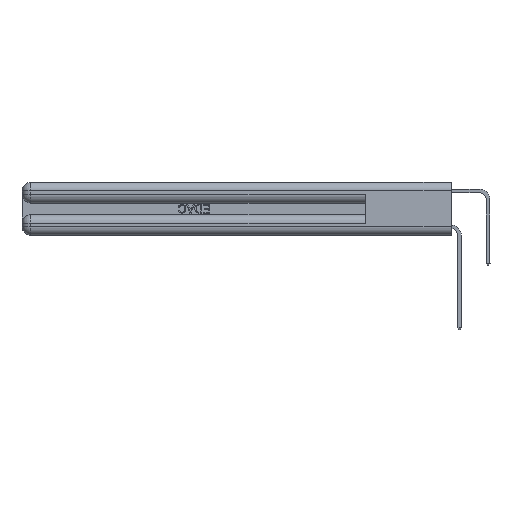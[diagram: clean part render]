
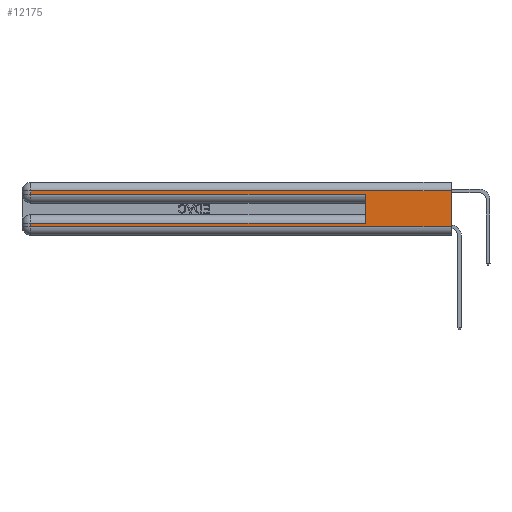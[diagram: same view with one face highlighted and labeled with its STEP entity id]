
A CAD part, left-side view. The second image highlights one B-rep face of the part: STEP entity #12175.
In plain terms, the highlighted planar face has unit normal (-1, 0, 0).
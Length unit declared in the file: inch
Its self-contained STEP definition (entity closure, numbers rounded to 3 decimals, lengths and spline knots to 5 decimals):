
#326 = CARTESIAN_POINT ( 'NONE',  ( 0., 0., 0.31 ) ) ;
#1134 = DIRECTION ( 'NONE',  ( 0., 1., 0. ) ) ;
#1836 = DIRECTION ( 'NONE',  ( 1., 0., 0. ) ) ;
#1907 = CARTESIAN_POINT ( 'NONE',  ( 0., 0., 0.285 ) ) ;
#2095 = DIRECTION ( 'NONE',  ( 0., -1., 0. ) ) ;
#2141 = EDGE_CURVE ( 'NONE', #10791, #7032, #10355, .T. ) ;
#2217 = DIRECTION ( 'NONE',  ( 0., 0., -1. ) ) ;
#2990 = EDGE_CURVE ( 'NONE', #7032, #5058, #13980, .T. ) ;
#3589 = VECTOR ( 'NONE', #2095, 39.37008 ) ;
#4436 = LINE ( 'NONE', #5590, #25466 ) ;
#4993 = DIRECTION ( 'NONE',  ( 0., 1., 0. ) ) ;
#5058 = VERTEX_POINT ( 'NONE', #28188 ) ;
#5516 = CARTESIAN_POINT ( 'NONE',  ( 0., 2.94, 0.31 ) ) ;
#5590 = CARTESIAN_POINT ( 'NONE',  ( 0., 0., 0.37 ) ) ;
#6096 = VECTOR ( 'NONE', #16822, 39.37008 ) ;
#6223 = CARTESIAN_POINT ( 'NONE',  ( 0., 0., 0.085 ) ) ;
#6437 = CARTESIAN_POINT ( 'NONE',  ( 0., 2.94, 0.37 ) ) ;
#7032 = VERTEX_POINT ( 'NONE', #15955 ) ;
#7646 = EDGE_CURVE ( 'NONE', #36003, #35059, #4436, .T. ) ;
#8826 = VERTEX_POINT ( 'NONE', #36131 ) ;
#9264 = AXIS2_PLACEMENT_3D ( 'NONE', #37642, #1836, #2217 ) ;
#10306 = EDGE_CURVE ( 'NONE', #36003, #10791, #22664, .T. ) ;
#10355 = LINE ( 'NONE', #13095, #13495 ) ;
#10791 = VERTEX_POINT ( 'NONE', #5516 ) ;
#11388 = LINE ( 'NONE', #37844, #6096 ) ;
#11722 = DIRECTION ( 'NONE',  ( 0., 0., -1. ) ) ;
#11881 = ORIENTED_EDGE ( 'NONE', *, *, #12666, .T. ) ;
#11940 = ORIENTED_EDGE ( 'NONE', *, *, #2990, .T. ) ;
#12175 = ADVANCED_FACE ( 'NONE', ( #31602 ), #37827, .F. ) ;
#12250 = ORIENTED_EDGE ( 'NONE', *, *, #2141, .T. ) ;
#12666 = EDGE_CURVE ( 'NONE', #25055, #29260, #32144, .T. ) ;
#13095 = CARTESIAN_POINT ( 'NONE',  ( 0., 2.94, 0.37 ) ) ;
#13495 = VECTOR ( 'NONE', #28443, 39.37008 ) ;
#13626 = VECTOR ( 'NONE', #11722, 39.37008 ) ;
#13885 = ORIENTED_EDGE ( 'NONE', *, *, #32631, .F. ) ;
#13980 = LINE ( 'NONE', #1907, #3589 ) ;
#15031 = ORIENTED_EDGE ( 'NONE', *, *, #7646, .F. ) ;
#15081 = ORIENTED_EDGE ( 'NONE', *, *, #21489, .T. ) ;
#15357 = LINE ( 'NONE', #6223, #29559 ) ;
#15955 = CARTESIAN_POINT ( 'NONE',  ( 0., 2.94, 0.285 ) ) ;
#16266 = ORIENTED_EDGE ( 'NONE', *, *, #10306, .T. ) ;
#16822 = DIRECTION ( 'NONE',  ( 0., -1., 0. ) ) ;
#16858 = VECTOR ( 'NONE', #4993, 39.37008 ) ;
#18440 = CARTESIAN_POINT ( 'NONE',  ( 0., 2.94, 0.06 ) ) ;
#18665 = CARTESIAN_POINT ( 'NONE',  ( 0., 0.6, 0.145 ) ) ;
#18967 = VECTOR ( 'NONE', #24479, 39.37008 ) ;
#19950 = DIRECTION ( 'NONE',  ( 0., 0., -1. ) ) ;
#20240 = CARTESIAN_POINT ( 'NONE',  ( 0., 0., 0.06 ) ) ;
#21489 = EDGE_CURVE ( 'NONE', #29260, #35059, #11388, .T. ) ;
#22183 = EDGE_CURVE ( 'NONE', #8826, #25055, #15357, .T. ) ;
#22352 = ORIENTED_EDGE ( 'NONE', *, *, #22183, .T. ) ;
#22664 = LINE ( 'NONE', #34963, #16858 ) ;
#22894 = CARTESIAN_POINT ( 'NONE',  ( 0., 2.94, 0.085 ) ) ;
#24479 = DIRECTION ( 'NONE',  ( 0., 0., 1. ) ) ;
#25055 = VERTEX_POINT ( 'NONE', #22894 ) ;
#25059 = LINE ( 'NONE', #18665, #18967 ) ;
#25466 = VECTOR ( 'NONE', #19950, 39.37008 ) ;
#28188 = CARTESIAN_POINT ( 'NONE',  ( 0., 0.6, 0.285 ) ) ;
#28443 = DIRECTION ( 'NONE',  ( 0., 0., -1. ) ) ;
#29260 = VERTEX_POINT ( 'NONE', #18440 ) ;
#29524 = EDGE_LOOP ( 'NONE', ( #15031, #16266, #12250, #11940, #13885, #22352, #11881, #15081 ) ) ;
#29559 = VECTOR ( 'NONE', #1134, 39.37008 ) ;
#31602 = FACE_OUTER_BOUND ( 'NONE', #29524, .T. ) ;
#32144 = LINE ( 'NONE', #6437, #13626 ) ;
#32631 = EDGE_CURVE ( 'NONE', #8826, #5058, #25059, .T. ) ;
#34963 = CARTESIAN_POINT ( 'NONE',  ( 0., 0., 0.31 ) ) ;
#35059 = VERTEX_POINT ( 'NONE', #20240 ) ;
#36003 = VERTEX_POINT ( 'NONE', #326 ) ;
#36131 = CARTESIAN_POINT ( 'NONE',  ( 0., 0.6, 0.085 ) ) ;
#37642 = CARTESIAN_POINT ( 'NONE',  ( 0., 0., 0.37 ) ) ;
#37827 = PLANE ( 'NONE',  #9264 ) ;
#37844 = CARTESIAN_POINT ( 'NONE',  ( 0., 0., 0.06 ) ) ;
